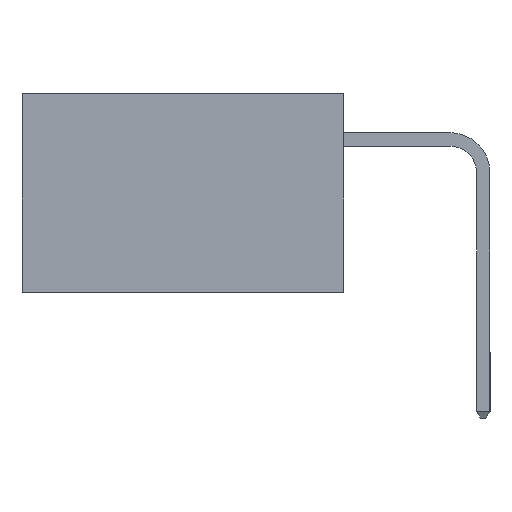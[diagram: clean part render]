
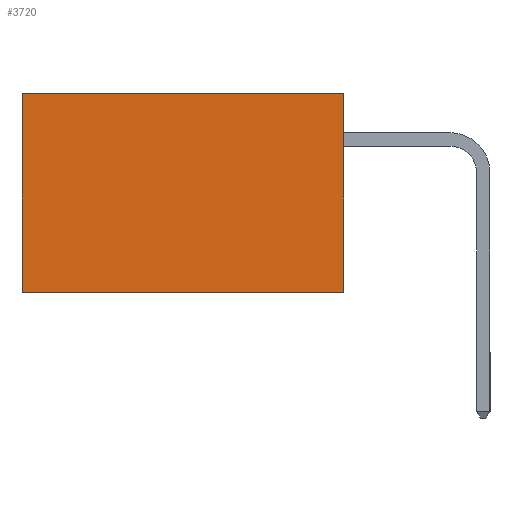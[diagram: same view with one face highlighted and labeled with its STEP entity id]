
A CAD part, left-side view. The second image highlights one B-rep face of the part: STEP entity #3720.
In plain terms, the highlighted planar face has unit normal (-1, 0, 0).
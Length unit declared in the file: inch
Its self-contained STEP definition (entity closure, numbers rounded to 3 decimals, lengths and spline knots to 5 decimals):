
#68 = VECTOR ( 'NONE', #3779, 39.37008 ) ;
#2348 = ORIENTED_EDGE ( 'NONE', *, *, #7118, .F. ) ;
#2942 = CARTESIAN_POINT ( 'NONE',  ( 0.298, 0., 0. ) ) ;
#3008 = EDGE_CURVE ( 'NONE', #17022, #16090, #14856, .T. ) ;
#3215 = CARTESIAN_POINT ( 'NONE',  ( 0.298, 0.6, -0.37 ) ) ;
#3720 = ADVANCED_FACE ( 'NONE', ( #18228 ), #12333, .F. ) ;
#3779 = DIRECTION ( 'NONE',  ( 0., 1., 0. ) ) ;
#4946 = DIRECTION ( 'NONE',  ( 0., 0., -1. ) ) ;
#5683 = CARTESIAN_POINT ( 'NONE',  ( 0.298, 0., 0. ) ) ;
#7017 = VECTOR ( 'NONE', #9488, 39.37008 ) ;
#7118 = EDGE_CURVE ( 'NONE', #11595, #16090, #20345, .T. ) ;
#7664 = ORIENTED_EDGE ( 'NONE', *, *, #22145, .T. ) ;
#7818 = LINE ( 'NONE', #12476, #68 ) ;
#8838 = DIRECTION ( 'NONE',  ( 0., 1., 0. ) ) ;
#9011 = CARTESIAN_POINT ( 'NONE',  ( 0.298, 0.6, 0. ) ) ;
#9488 = DIRECTION ( 'NONE',  ( 0., 0., -1. ) ) ;
#11595 = VERTEX_POINT ( 'NONE', #20323 ) ;
#12333 = PLANE ( 'NONE',  #13886 ) ;
#12476 = CARTESIAN_POINT ( 'NONE',  ( 0.298, 0., 0. ) ) ;
#12738 = LINE ( 'NONE', #5683, #7017 ) ;
#13886 = AXIS2_PLACEMENT_3D ( 'NONE', #21568, #15939, #19438 ) ;
#14497 = ORIENTED_EDGE ( 'NONE', *, *, #3008, .T. ) ;
#14856 = LINE ( 'NONE', #23247, #20253 ) ;
#15007 = ORIENTED_EDGE ( 'NONE', *, *, #19309, .F. ) ;
#15939 = DIRECTION ( 'NONE',  ( 1., 0., 0. ) ) ;
#16090 = VERTEX_POINT ( 'NONE', #3215 ) ;
#16819 = VERTEX_POINT ( 'NONE', #2942 ) ;
#17022 = VERTEX_POINT ( 'NONE', #9011 ) ;
#17768 = CARTESIAN_POINT ( 'NONE',  ( 0.298, 0., -0.37 ) ) ;
#18228 = FACE_OUTER_BOUND ( 'NONE', #18901, .T. ) ;
#18901 = EDGE_LOOP ( 'NONE', ( #14497, #2348, #15007, #7664 ) ) ;
#19309 = EDGE_CURVE ( 'NONE', #16819, #11595, #12738, .T. ) ;
#19438 = DIRECTION ( 'NONE',  ( 0., 0., -1. ) ) ;
#19780 = VECTOR ( 'NONE', #8838, 39.37008 ) ;
#20253 = VECTOR ( 'NONE', #4946, 39.37008 ) ;
#20323 = CARTESIAN_POINT ( 'NONE',  ( 0.298, 0., -0.37 ) ) ;
#20345 = LINE ( 'NONE', #17768, #19780 ) ;
#21568 = CARTESIAN_POINT ( 'NONE',  ( 0.298, 0., 0. ) ) ;
#22145 = EDGE_CURVE ( 'NONE', #16819, #17022, #7818, .T. ) ;
#23247 = CARTESIAN_POINT ( 'NONE',  ( 0.298, 0.6, 0. ) ) ;
